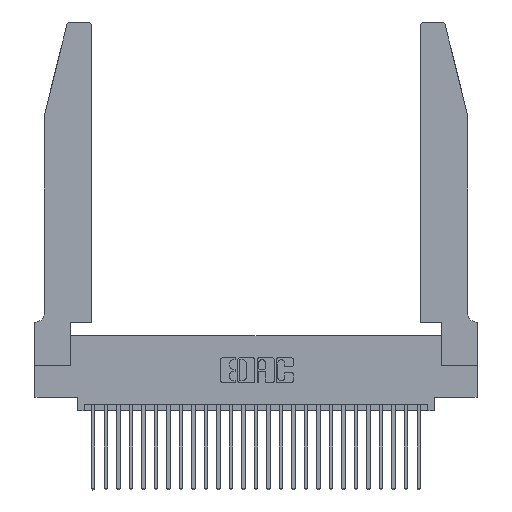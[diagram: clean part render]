
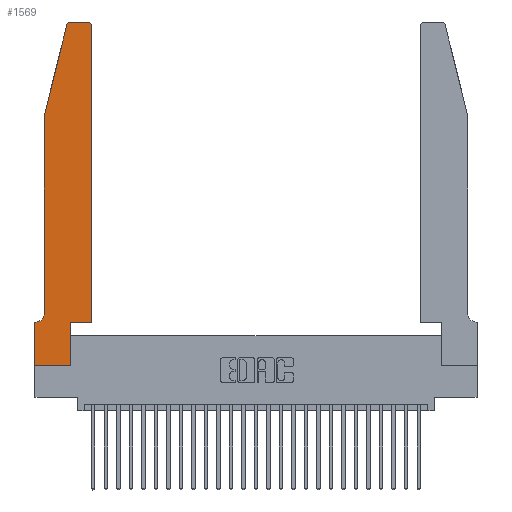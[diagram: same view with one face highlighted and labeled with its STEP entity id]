
A CAD part, top view. The second image highlights one B-rep face of the part: STEP entity #1569.
In plain terms, the highlighted planar face has unit normal (0, 0, 1).
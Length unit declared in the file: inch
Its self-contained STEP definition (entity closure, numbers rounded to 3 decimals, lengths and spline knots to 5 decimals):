
#15 = VERTEX_POINT ( 'NONE', #2215 ) ;
#119 = ORIENTED_EDGE ( 'NONE', *, *, #27073, .T. ) ;
#554 = EDGE_CURVE ( 'NONE', #19721, #13919, #3643, .T. ) ;
#1216 = PLANE ( 'NONE',  #24197 ) ;
#1516 = CARTESIAN_POINT ( 'NONE',  ( 0.4505, 2.72, 0.37 ) ) ;
#1569 = ADVANCED_FACE ( 'NONE', ( #21924 ), #1216, .T. ) ;
#1864 = CARTESIAN_POINT ( 'NONE',  ( 0., 0., 0.37 ) ) ;
#2215 = CARTESIAN_POINT ( 'NONE',  ( 0.2865, 0.35, 0.37 ) ) ;
#2791 = EDGE_CURVE ( 'NONE', #15, #26030, #24586, .T. ) ;
#3295 = LINE ( 'NONE', #3436, #10475 ) ;
#3337 = DIRECTION ( 'NONE',  ( -1., 0., 0. ) ) ;
#3436 = CARTESIAN_POINT ( 'NONE',  ( 0.0755, 0.35, 0.37 ) ) ;
#3643 = LINE ( 'NONE', #1864, #11148 ) ;
#4003 = DIRECTION ( 'NONE',  ( 1., 0., 0. ) ) ;
#4780 = VERTEX_POINT ( 'NONE', #5719 ) ;
#4929 = VECTOR ( 'NONE', #9801, 39.37008 ) ;
#5719 = CARTESIAN_POINT ( 'NONE',  ( 0.0755, 0.42, 0.37 ) ) ;
#6561 = VERTEX_POINT ( 'NONE', #11676 ) ;
#6861 = CARTESIAN_POINT ( 'NONE',  ( 0.0055, 0.42, 0.37 ) ) ;
#7209 = LINE ( 'NONE', #19873, #27178 ) ;
#8409 = VECTOR ( 'NONE', #16217, 39.37008 ) ;
#8514 = ORIENTED_EDGE ( 'NONE', *, *, #22676, .T. ) ;
#8752 = LINE ( 'NONE', #22316, #21576 ) ;
#8804 = DIRECTION ( 'NONE',  ( -1., 0., 0. ) ) ;
#9104 = CIRCLE ( 'NONE', #20909, 0.07 ) ;
#9203 = DIRECTION ( 'NONE',  ( 0., 1., 0. ) ) ;
#9623 = AXIS2_PLACEMENT_3D ( 'NONE', #13071, #28016, #19412 ) ;
#9801 = DIRECTION ( 'NONE',  ( -1., 0., 0. ) ) ;
#10152 = DIRECTION ( 'NONE',  ( -0.239, -0.971, 0. ) ) ;
#10349 = ORIENTED_EDGE ( 'NONE', *, *, #26826, .T. ) ;
#10475 = VECTOR ( 'NONE', #3337, 39.37008 ) ;
#10896 = EDGE_CURVE ( 'NONE', #27996, #22379, #21202, .T. ) ;
#11148 = VECTOR ( 'NONE', #25953, 39.37008 ) ;
#11392 = CARTESIAN_POINT ( 'NONE',  ( 0.0755, 2., 0.37 ) ) ;
#11676 = CARTESIAN_POINT ( 'NONE',  ( 0.284, 2.75, 0.37 ) ) ;
#12061 = CARTESIAN_POINT ( 'NONE',  ( 0.4505, 0.35, 0.37 ) ) ;
#12089 = DIRECTION ( 'NONE',  ( 0., 0., 1. ) ) ;
#12880 = DIRECTION ( 'NONE',  ( 0., -1., 0. ) ) ;
#13071 = CARTESIAN_POINT ( 'NONE',  ( 0.4205, 2.72, 0.37 ) ) ;
#13152 = CIRCLE ( 'NONE', #26328, 0.03 ) ;
#13418 = LINE ( 'NONE', #22843, #4929 ) ;
#13546 = EDGE_CURVE ( 'NONE', #13919, #15, #7209, .T. ) ;
#13766 = CARTESIAN_POINT ( 'NONE',  ( 0.0755, 2., 0.37 ) ) ;
#13919 = VERTEX_POINT ( 'NONE', #25515 ) ;
#14549 = ORIENTED_EDGE ( 'NONE', *, *, #13546, .T. ) ;
#14735 = ORIENTED_EDGE ( 'NONE', *, *, #27031, .T. ) ;
#14838 = DIRECTION ( 'NONE',  ( 0., 0., 1. ) ) ;
#16217 = DIRECTION ( 'NONE',  ( 0., -1., 0. ) ) ;
#16747 = EDGE_CURVE ( 'NONE', #26030, #16978, #8752, .T. ) ;
#16811 = ORIENTED_EDGE ( 'NONE', *, *, #2791, .T. ) ;
#16950 = CARTESIAN_POINT ( 'NONE',  ( 0.25487, 2.72718, 0.37 ) ) ;
#16978 = VERTEX_POINT ( 'NONE', #1516 ) ;
#17132 = CARTESIAN_POINT ( 'NONE',  ( 0., 0., 0.37 ) ) ;
#17139 = VERTEX_POINT ( 'NONE', #25975 ) ;
#17659 = ORIENTED_EDGE ( 'NONE', *, *, #23598, .T. ) ;
#17963 = VERTEX_POINT ( 'NONE', #20346 ) ;
#18271 = EDGE_LOOP ( 'NONE', ( #24925, #14735, #22713, #17659, #119, #10349, #18523, #26607, #14549, #16811, #20341, #8514 ) ) ;
#18523 = ORIENTED_EDGE ( 'NONE', *, *, #22682, .T. ) ;
#18537 = LINE ( 'NONE', #17132, #22989 ) ;
#18608 = CARTESIAN_POINT ( 'NONE',  ( 0., 0., 0.37 ) ) ;
#19363 = CARTESIAN_POINT ( 'NONE',  ( 0.284, 2.72, 0.37 ) ) ;
#19412 = DIRECTION ( 'NONE',  ( 1., 0., 0. ) ) ;
#19721 = VERTEX_POINT ( 'NONE', #18608 ) ;
#19873 = CARTESIAN_POINT ( 'NONE',  ( 0.2865, 0.35, 0.37 ) ) ;
#20341 = ORIENTED_EDGE ( 'NONE', *, *, #16747, .T. ) ;
#20346 = CARTESIAN_POINT ( 'NONE',  ( 0.4205, 2.75, 0.37 ) ) ;
#20677 = CARTESIAN_POINT ( 'NONE',  ( 0., 0.35, 0.37 ) ) ;
#20851 = VECTOR ( 'NONE', #10152, 39.37008 ) ;
#20885 = LINE ( 'NONE', #13766, #8409 ) ;
#20909 = AXIS2_PLACEMENT_3D ( 'NONE', #6861, #21916, #8804 ) ;
#21043 = DIRECTION ( 'NONE',  ( 1., 0., 0. ) ) ;
#21202 = LINE ( 'NONE', #11392, #20851 ) ;
#21287 = CIRCLE ( 'NONE', #9623, 0.03 ) ;
#21416 = DIRECTION ( 'NONE',  ( 1., 0., 0. ) ) ;
#21576 = VECTOR ( 'NONE', #22791, 39.37008 ) ;
#21916 = DIRECTION ( 'NONE',  ( 0., 0., -1. ) ) ;
#21924 = FACE_OUTER_BOUND ( 'NONE', #18271, .T. ) ;
#21925 = VERTEX_POINT ( 'NONE', #23752 ) ;
#22316 = CARTESIAN_POINT ( 'NONE',  ( 0.4505, 0.35, 0.37 ) ) ;
#22379 = VERTEX_POINT ( 'NONE', #24983 ) ;
#22676 = EDGE_CURVE ( 'NONE', #16978, #17963, #21287, .T. ) ;
#22682 = EDGE_CURVE ( 'NONE', #21925, #19721, #18537, .T. ) ;
#22713 = ORIENTED_EDGE ( 'NONE', *, *, #10896, .T. ) ;
#22791 = DIRECTION ( 'NONE',  ( 0., 1., 0. ) ) ;
#22843 = CARTESIAN_POINT ( 'NONE',  ( 0.2605, 2.75, 0.37 ) ) ;
#22989 = VECTOR ( 'NONE', #12880, 39.37008 ) ;
#23598 = EDGE_CURVE ( 'NONE', #22379, #4780, #20885, .T. ) ;
#23752 = CARTESIAN_POINT ( 'NONE',  ( 0., 0.35, 0.37 ) ) ;
#24041 = EDGE_CURVE ( 'NONE', #17963, #6561, #13418, .T. ) ;
#24197 = AXIS2_PLACEMENT_3D ( 'NONE', #20677, #12089, #21043 ) ;
#24586 = LINE ( 'NONE', #25002, #26272 ) ;
#24925 = ORIENTED_EDGE ( 'NONE', *, *, #24041, .T. ) ;
#24983 = CARTESIAN_POINT ( 'NONE',  ( 0.0755, 2., 0.37 ) ) ;
#25002 = CARTESIAN_POINT ( 'NONE',  ( 0.4505, 0.35, 0.37 ) ) ;
#25515 = CARTESIAN_POINT ( 'NONE',  ( 0.2865, 0., 0.37 ) ) ;
#25953 = DIRECTION ( 'NONE',  ( 1., 0., 0. ) ) ;
#25975 = CARTESIAN_POINT ( 'NONE',  ( 0.0055, 0.35, 0.37 ) ) ;
#26030 = VERTEX_POINT ( 'NONE', #12061 ) ;
#26272 = VECTOR ( 'NONE', #21416, 39.37008 ) ;
#26328 = AXIS2_PLACEMENT_3D ( 'NONE', #19363, #14838, #4003 ) ;
#26607 = ORIENTED_EDGE ( 'NONE', *, *, #554, .T. ) ;
#26826 = EDGE_CURVE ( 'NONE', #17139, #21925, #3295, .T. ) ;
#27031 = EDGE_CURVE ( 'NONE', #6561, #27996, #13152, .T. ) ;
#27073 = EDGE_CURVE ( 'NONE', #4780, #17139, #9104, .T. ) ;
#27178 = VECTOR ( 'NONE', #9203, 39.37008 ) ;
#27996 = VERTEX_POINT ( 'NONE', #16950 ) ;
#28016 = DIRECTION ( 'NONE',  ( 0., 0., 1. ) ) ;
